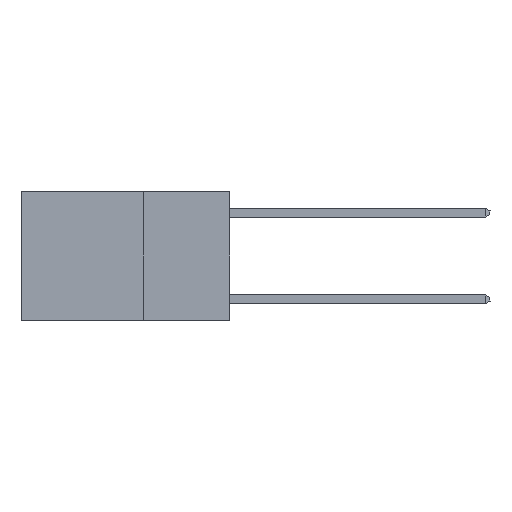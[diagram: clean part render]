
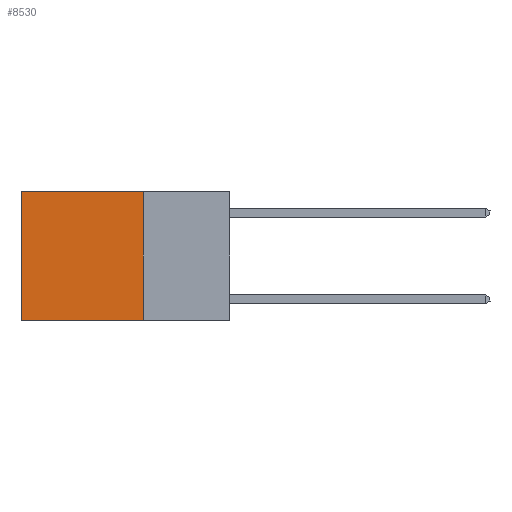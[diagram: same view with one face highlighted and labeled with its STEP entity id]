
A CAD part, left-side view. The second image highlights one B-rep face of the part: STEP entity #8530.
In plain terms, the highlighted planar face has unit normal (-1, 0, 0).
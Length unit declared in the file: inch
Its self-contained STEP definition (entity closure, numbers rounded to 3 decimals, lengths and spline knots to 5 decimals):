
#26 = LINE ( 'NONE', #1646, #2714 ) ;
#1066 = ORIENTED_EDGE ( 'NONE', *, *, #20072, .T. ) ;
#1646 = CARTESIAN_POINT ( 'NONE',  ( 0.2625, 0.25, 0. ) ) ;
#2295 = VERTEX_POINT ( 'NONE', #13596 ) ;
#2714 = VECTOR ( 'NONE', #18982, 39.37008 ) ;
#2837 = EDGE_CURVE ( 'NONE', #2295, #8665, #22553, .T. ) ;
#3265 = VERTEX_POINT ( 'NONE', #20692 ) ;
#5116 = LINE ( 'NONE', #21317, #15793 ) ;
#6095 = EDGE_CURVE ( 'NONE', #12000, #8665, #19094, .T. ) ;
#6366 = FACE_OUTER_BOUND ( 'NONE', #8956, .T. ) ;
#6589 = DIRECTION ( 'NONE',  ( 0., 0., -1. ) ) ;
#7327 = ORIENTED_EDGE ( 'NONE', *, *, #21806, .F. ) ;
#7693 = CARTESIAN_POINT ( 'NONE',  ( 0.2625, 0.25, -0.37 ) ) ;
#7812 = VECTOR ( 'NONE', #12831, 39.37008 ) ;
#8318 = CARTESIAN_POINT ( 'NONE',  ( 0.2625, 0.6, 0. ) ) ;
#8530 = ADVANCED_FACE ( 'NONE', ( #6366 ), #15067, .F. ) ;
#8665 = VERTEX_POINT ( 'NONE', #18552 ) ;
#8956 = EDGE_LOOP ( 'NONE', ( #15690, #22006, #7327, #1066 ) ) ;
#10019 = DIRECTION ( 'NONE',  ( 1., 0., 0. ) ) ;
#10156 = CARTESIAN_POINT ( 'NONE',  ( 0.2625, 0.25, -0.37 ) ) ;
#11863 = DIRECTION ( 'NONE',  ( 0., 1., 0. ) ) ;
#12000 = VERTEX_POINT ( 'NONE', #10156 ) ;
#12831 = DIRECTION ( 'NONE',  ( 0., 1., 0. ) ) ;
#13596 = CARTESIAN_POINT ( 'NONE',  ( 0.2625, 0.6, 0. ) ) ;
#15067 = PLANE ( 'NONE',  #18112 ) ;
#15690 = ORIENTED_EDGE ( 'NONE', *, *, #2837, .T. ) ;
#15793 = VECTOR ( 'NONE', #11863, 39.37008 ) ;
#17034 = DIRECTION ( 'NONE',  ( 0., 0., -1. ) ) ;
#18112 = AXIS2_PLACEMENT_3D ( 'NONE', #18772, #10019, #17034 ) ;
#18552 = CARTESIAN_POINT ( 'NONE',  ( 0.2625, 0.6, -0.37 ) ) ;
#18662 = VECTOR ( 'NONE', #6589, 39.37008 ) ;
#18772 = CARTESIAN_POINT ( 'NONE',  ( 0.2625, 0.25, 0. ) ) ;
#18982 = DIRECTION ( 'NONE',  ( 0., 0., -1. ) ) ;
#19094 = LINE ( 'NONE', #7693, #7812 ) ;
#20072 = EDGE_CURVE ( 'NONE', #3265, #2295, #5116, .T. ) ;
#20692 = CARTESIAN_POINT ( 'NONE',  ( 0.2625, 0.25, 0. ) ) ;
#21317 = CARTESIAN_POINT ( 'NONE',  ( 0.2625, 0.25, 0. ) ) ;
#21806 = EDGE_CURVE ( 'NONE', #3265, #12000, #26, .T. ) ;
#22006 = ORIENTED_EDGE ( 'NONE', *, *, #6095, .F. ) ;
#22553 = LINE ( 'NONE', #8318, #18662 ) ;
